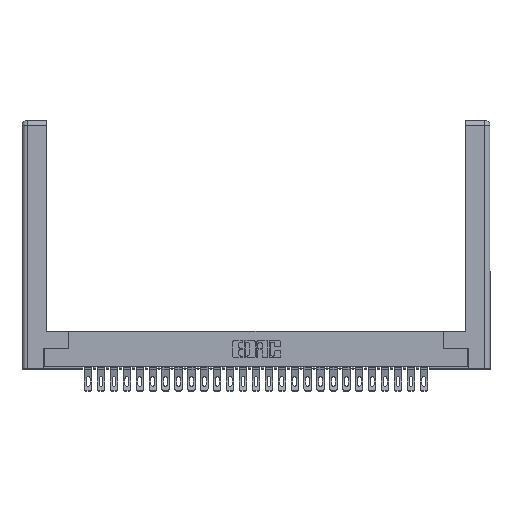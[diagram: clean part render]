
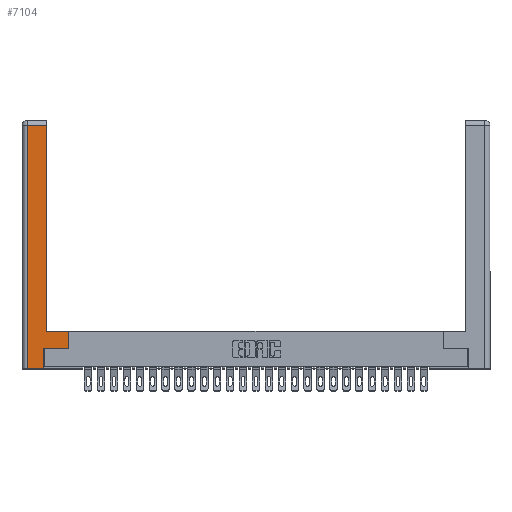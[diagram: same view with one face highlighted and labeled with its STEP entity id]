
A CAD part, top view. The second image highlights one B-rep face of the part: STEP entity #7104.
In plain terms, the highlighted planar face has unit normal (0, 0, 1).
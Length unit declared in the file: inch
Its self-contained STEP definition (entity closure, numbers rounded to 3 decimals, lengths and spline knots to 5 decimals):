
#323 = EDGE_CURVE ( 'NONE', #11431, #24678, #20630, .T. ) ;
#3418 = ORIENTED_EDGE ( 'NONE', *, *, #17760, .T. ) ;
#3627 = EDGE_CURVE ( 'NONE', #24678, #11387, #22455, .T. ) ;
#4141 = CARTESIAN_POINT ( 'NONE',  ( 0.0615, 0., 0. ) ) ;
#5858 = ORIENTED_EDGE ( 'NONE', *, *, #9365, .T. ) ;
#6279 = EDGE_CURVE ( 'NONE', #11877, #14392, #27269, .T. ) ;
#6468 = VECTOR ( 'NONE', #8105, 39.37008 ) ;
#6546 = ORIENTED_EDGE ( 'NONE', *, *, #6279, .T. ) ;
#6734 = VERTEX_POINT ( 'NONE', #26756 ) ;
#7104 = ADVANCED_FACE ( 'NONE', ( #34282 ), #14099, .F. ) ;
#7683 = VECTOR ( 'NONE', #29202, 39.37008 ) ;
#8105 = DIRECTION ( 'NONE',  ( 1., 0., 0. ) ) ;
#8208 = VERTEX_POINT ( 'NONE', #21871 ) ;
#8358 = CARTESIAN_POINT ( 'NONE',  ( 0.295, 2.94, 0. ) ) ;
#8476 = DIRECTION ( 'NONE',  ( 0., 1., 0. ) ) ;
#9365 = EDGE_CURVE ( 'NONE', #34008, #11877, #33277, .T. ) ;
#9450 = DIRECTION ( 'NONE',  ( -1., 0., 0. ) ) ;
#9701 = VECTOR ( 'NONE', #29295, 39.37008 ) ;
#9738 = LINE ( 'NONE', #18160, #7683 ) ;
#10298 = CARTESIAN_POINT ( 'NONE',  ( 0.565, 0.45, 0. ) ) ;
#10477 = LINE ( 'NONE', #10298, #15882 ) ;
#10543 = EDGE_CURVE ( 'NONE', #6734, #11431, #29501, .T. ) ;
#10637 = ORIENTED_EDGE ( 'NONE', *, *, #18262, .T. ) ;
#11387 = VERTEX_POINT ( 'NONE', #29785 ) ;
#11431 = VERTEX_POINT ( 'NONE', #4141 ) ;
#11533 = CARTESIAN_POINT ( 'NONE',  ( 0.265, 0., 0. ) ) ;
#11877 = VERTEX_POINT ( 'NONE', #31809 ) ;
#13154 = ORIENTED_EDGE ( 'NONE', *, *, #10543, .T. ) ;
#13961 = ORIENTED_EDGE ( 'NONE', *, *, #28568, .T. ) ;
#14099 = PLANE ( 'NONE',  #16596 ) ;
#14392 = VERTEX_POINT ( 'NONE', #8358 ) ;
#15536 = DIRECTION ( 'NONE',  ( -1., 0., 0. ) ) ;
#15882 = VECTOR ( 'NONE', #31537, 39.37008 ) ;
#16596 = AXIS2_PLACEMENT_3D ( 'NONE', #19001, #17479, #9450 ) ;
#17479 = DIRECTION ( 'NONE',  ( 0., 0., -1. ) ) ;
#17760 = EDGE_CURVE ( 'NONE', #11387, #8208, #9738, .T. ) ;
#18160 = CARTESIAN_POINT ( 'NONE',  ( 0.565, 0.245, 0. ) ) ;
#18262 = EDGE_CURVE ( 'NONE', #14392, #6734, #33377, .T. ) ;
#18861 = CARTESIAN_POINT ( 'NONE',  ( 0.565, 0.45, 0. ) ) ;
#19001 = CARTESIAN_POINT ( 'NONE',  ( 0., 0., 0. ) ) ;
#19132 = EDGE_LOOP ( 'NONE', ( #6546, #10637, #13154, #19138, #22113, #3418, #13961, #5858 ) ) ;
#19138 = ORIENTED_EDGE ( 'NONE', *, *, #323, .T. ) ;
#19186 = VECTOR ( 'NONE', #15536, 39.37008 ) ;
#20630 = LINE ( 'NONE', #21473, #6468 ) ;
#21473 = CARTESIAN_POINT ( 'NONE',  ( 0.265, 0., 0. ) ) ;
#21871 = CARTESIAN_POINT ( 'NONE',  ( 0.565, 0.245, 0. ) ) ;
#22113 = ORIENTED_EDGE ( 'NONE', *, *, #3627, .T. ) ;
#22455 = LINE ( 'NONE', #24428, #30723 ) ;
#24428 = CARTESIAN_POINT ( 'NONE',  ( 0.265, 0.245, 0. ) ) ;
#24678 = VERTEX_POINT ( 'NONE', #11533 ) ;
#25931 = CARTESIAN_POINT ( 'NONE',  ( 0.0615, 0., 0. ) ) ;
#26437 = VECTOR ( 'NONE', #32242, 39.37008 ) ;
#26756 = CARTESIAN_POINT ( 'NONE',  ( 0.0615, 2.94, 0. ) ) ;
#27269 = LINE ( 'NONE', #31678, #26437 ) ;
#27302 = CARTESIAN_POINT ( 'NONE',  ( 0.295, 0.45, 0. ) ) ;
#28250 = VECTOR ( 'NONE', #28579, 39.37008 ) ;
#28568 = EDGE_CURVE ( 'NONE', #8208, #34008, #10477, .T. ) ;
#28579 = DIRECTION ( 'NONE',  ( 0., -1., 0. ) ) ;
#29202 = DIRECTION ( 'NONE',  ( 1., 0., 0. ) ) ;
#29295 = DIRECTION ( 'NONE',  ( -1., 0., 0. ) ) ;
#29501 = LINE ( 'NONE', #25931, #28250 ) ;
#29785 = CARTESIAN_POINT ( 'NONE',  ( 0.265, 0.245, 0. ) ) ;
#30723 = VECTOR ( 'NONE', #8476, 39.37008 ) ;
#31537 = DIRECTION ( 'NONE',  ( 0., 1., 0. ) ) ;
#31678 = CARTESIAN_POINT ( 'NONE',  ( 0.295, 3., 0. ) ) ;
#31697 = CARTESIAN_POINT ( 'NONE',  ( 0.0615, 2.94, 0. ) ) ;
#31809 = CARTESIAN_POINT ( 'NONE',  ( 0.295, 0.45, 0. ) ) ;
#32242 = DIRECTION ( 'NONE',  ( 0., 1., 0. ) ) ;
#33277 = LINE ( 'NONE', #27302, #19186 ) ;
#33377 = LINE ( 'NONE', #31697, #9701 ) ;
#34008 = VERTEX_POINT ( 'NONE', #18861 ) ;
#34282 = FACE_OUTER_BOUND ( 'NONE', #19132, .T. ) ;
